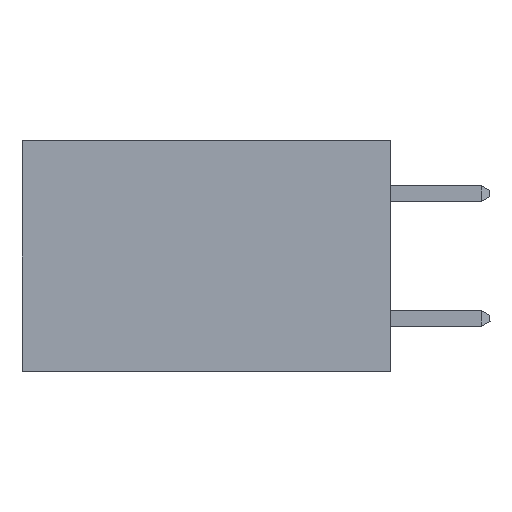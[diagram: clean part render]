
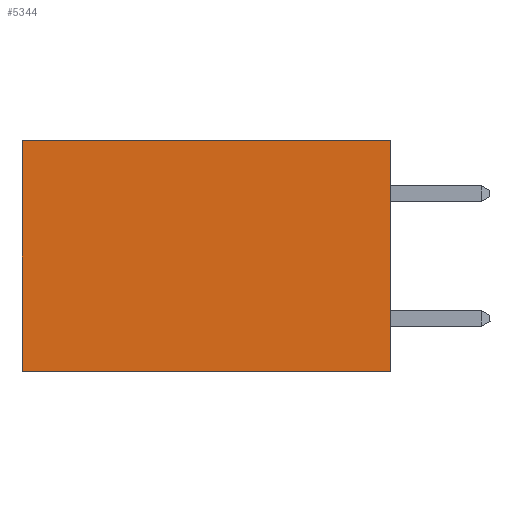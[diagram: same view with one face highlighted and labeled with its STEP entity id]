
A CAD part, left-side view. The second image highlights one B-rep face of the part: STEP entity #5344.
In plain terms, the highlighted planar face has unit normal (-1, 0, 0).
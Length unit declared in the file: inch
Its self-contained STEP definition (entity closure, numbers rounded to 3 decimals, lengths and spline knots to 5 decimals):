
#1911 = VERTEX_POINT ( 'NONE', #25961 ) ;
#2699 = EDGE_LOOP ( 'NONE', ( #16781, #11116, #26060, #15636 ) ) ;
#3080 = CARTESIAN_POINT ( 'NONE',  ( 0.277, 0.59, -0.37 ) ) ;
#3104 = DIRECTION ( 'NONE',  ( 0., 1., 0. ) ) ;
#3350 = EDGE_CURVE ( 'NONE', #1911, #16860, #13208, .T. ) ;
#5344 = ADVANCED_FACE ( 'NONE', ( #14700 ), #15401, .F. ) ;
#7197 = CARTESIAN_POINT ( 'NONE',  ( 0.277, 0., -0.37 ) ) ;
#7881 = DIRECTION ( 'NONE',  ( 0., 0., -1. ) ) ;
#8104 = CARTESIAN_POINT ( 'NONE',  ( 0.277, 0., -0.37 ) ) ;
#8443 = CARTESIAN_POINT ( 'NONE',  ( 0.277, 0., -0.37 ) ) ;
#9283 = DIRECTION ( 'NONE',  ( 1., 0., 0. ) ) ;
#9823 = VECTOR ( 'NONE', #21815, 39.37008 ) ;
#9980 = CARTESIAN_POINT ( 'NONE',  ( 0.277, 0.59, 0. ) ) ;
#10971 = AXIS2_PLACEMENT_3D ( 'NONE', #7197, #9283, #23571 ) ;
#11116 = ORIENTED_EDGE ( 'NONE', *, *, #15930, .F. ) ;
#11639 = VERTEX_POINT ( 'NONE', #3080 ) ;
#12266 = DIRECTION ( 'NONE',  ( 0., 1., 0. ) ) ;
#13208 = LINE ( 'NONE', #8443, #24040 ) ;
#13209 = CARTESIAN_POINT ( 'NONE',  ( 0.277, 0., -0.37 ) ) ;
#13271 = LINE ( 'NONE', #23681, #18111 ) ;
#14700 = FACE_OUTER_BOUND ( 'NONE', #2699, .T. ) ;
#15231 = LINE ( 'NONE', #8104, #25398 ) ;
#15401 = PLANE ( 'NONE',  #10971 ) ;
#15636 = ORIENTED_EDGE ( 'NONE', *, *, #21284, .T. ) ;
#15930 = EDGE_CURVE ( 'NONE', #16860, #11639, #15231, .T. ) ;
#15934 = LINE ( 'NONE', #25910, #9823 ) ;
#16781 = ORIENTED_EDGE ( 'NONE', *, *, #19899, .T. ) ;
#16860 = VERTEX_POINT ( 'NONE', #13209 ) ;
#18111 = VECTOR ( 'NONE', #3104, 39.37008 ) ;
#19899 = EDGE_CURVE ( 'NONE', #22692, #11639, #15934, .T. ) ;
#21284 = EDGE_CURVE ( 'NONE', #1911, #22692, #13271, .T. ) ;
#21815 = DIRECTION ( 'NONE',  ( 0., 0., -1. ) ) ;
#22692 = VERTEX_POINT ( 'NONE', #9980 ) ;
#23571 = DIRECTION ( 'NONE',  ( 0., 0., -1. ) ) ;
#23681 = CARTESIAN_POINT ( 'NONE',  ( 0.277, 0., 0. ) ) ;
#24040 = VECTOR ( 'NONE', #7881, 39.37008 ) ;
#25398 = VECTOR ( 'NONE', #12266, 39.37008 ) ;
#25910 = CARTESIAN_POINT ( 'NONE',  ( 0.277, 0.59, -0.37 ) ) ;
#25961 = CARTESIAN_POINT ( 'NONE',  ( 0.277, 0., 0. ) ) ;
#26060 = ORIENTED_EDGE ( 'NONE', *, *, #3350, .F. ) ;
